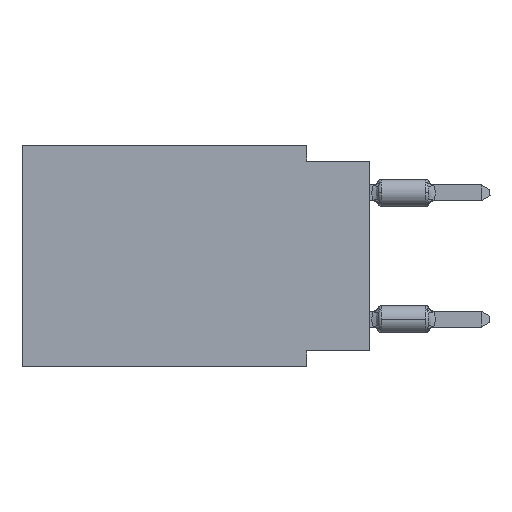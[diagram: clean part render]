
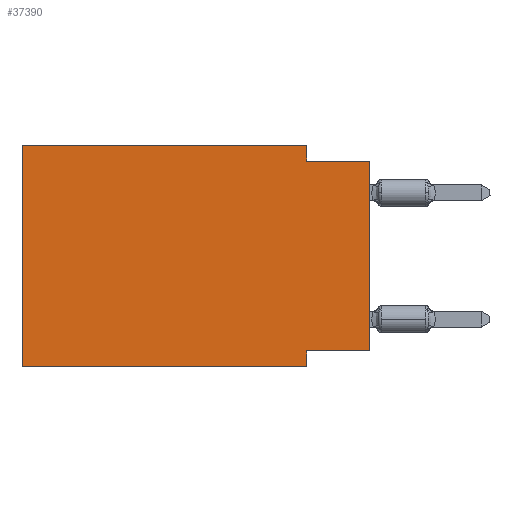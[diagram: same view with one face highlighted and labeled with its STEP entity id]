
A CAD part, left-side view. The second image highlights one B-rep face of the part: STEP entity #37390.
In plain terms, the highlighted planar face has unit normal (-1, 0, 0).
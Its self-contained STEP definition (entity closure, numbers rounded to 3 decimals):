
#150 = CARTESIAN_POINT ( 'NONE',  ( 0., 13.97, 0. ) ) ;
#561 = LINE ( 'NONE', #11217, #10341 ) ;
#792 = DIRECTION ( 'NONE',  ( 0., 0., -1. ) ) ;
#1008 = VERTEX_POINT ( 'NONE', #30699 ) ;
#1173 = DIRECTION ( 'NONE',  ( 0., 0., -1. ) ) ;
#2580 = LINE ( 'NONE', #2829, #40246 ) ;
#2829 = CARTESIAN_POINT ( 'NONE',  ( 0., 13.97, 0. ) ) ;
#3080 = ORIENTED_EDGE ( 'NONE', *, *, #45692, .F. ) ;
#5302 = CARTESIAN_POINT ( 'NONE',  ( 0., 0., 0. ) ) ;
#5452 = ORIENTED_EDGE ( 'NONE', *, *, #14774, .F. ) ;
#6140 = ORIENTED_EDGE ( 'NONE', *, *, #12411, .F. ) ;
#8449 = VECTOR ( 'NONE', #9900, 1000. ) ;
#8931 = AXIS2_PLACEMENT_3D ( 'NONE', #49040, #38356, #45553 ) ;
#9270 = LINE ( 'NONE', #20926, #18424 ) ;
#9900 = DIRECTION ( 'NONE',  ( 0., -1., 0. ) ) ;
#10341 = VECTOR ( 'NONE', #792, 1000. ) ;
#11217 = CARTESIAN_POINT ( 'NONE',  ( 0., 2.54, -8.89 ) ) ;
#12357 = LINE ( 'NONE', #23748, #25128 ) ;
#12411 = EDGE_CURVE ( 'NONE', #19675, #39759, #42293, .T. ) ;
#13213 = VERTEX_POINT ( 'NONE', #41444 ) ;
#13429 = VECTOR ( 'NONE', #1173, 1000. ) ;
#14661 = EDGE_CURVE ( 'NONE', #21927, #38828, #38777, .T. ) ;
#14774 = EDGE_CURVE ( 'NONE', #21927, #41085, #9270, .T. ) ;
#15375 = ORIENTED_EDGE ( 'NONE', *, *, #14661, .T. ) ;
#17890 = CARTESIAN_POINT ( 'NONE',  ( 0., 13.97, 0. ) ) ;
#18424 = VECTOR ( 'NONE', #43947, 1000. ) ;
#18802 = FACE_OUTER_BOUND ( 'NONE', #39040, .T. ) ;
#19052 = ORIENTED_EDGE ( 'NONE', *, *, #45977, .T. ) ;
#19507 = ORIENTED_EDGE ( 'NONE', *, *, #26186, .F. ) ;
#19675 = VERTEX_POINT ( 'NONE', #17890 ) ;
#20926 = CARTESIAN_POINT ( 'NONE',  ( 0., 0., -8.255 ) ) ;
#21653 = CARTESIAN_POINT ( 'NONE',  ( 0., 0., -0.635 ) ) ;
#21927 = VERTEX_POINT ( 'NONE', #41802 ) ;
#23737 = LINE ( 'NONE', #38854, #13429 ) ;
#23748 = CARTESIAN_POINT ( 'NONE',  ( 0., 13.97, -8.89 ) ) ;
#25128 = VECTOR ( 'NONE', #30941, 1000. ) ;
#26145 = VECTOR ( 'NONE', #26931, 1000. ) ;
#26186 = EDGE_CURVE ( 'NONE', #13213, #19675, #2580, .T. ) ;
#26931 = DIRECTION ( 'NONE',  ( 0., -1., 0. ) ) ;
#27170 = EDGE_CURVE ( 'NONE', #41085, #1008, #561, .T. ) ;
#27893 = ORIENTED_EDGE ( 'NONE', *, *, #28112, .F. ) ;
#28112 = EDGE_CURVE ( 'NONE', #39759, #28387, #23737, .T. ) ;
#28387 = VERTEX_POINT ( 'NONE', #45194 ) ;
#30433 = PLANE ( 'NONE',  #8931 ) ;
#30699 = CARTESIAN_POINT ( 'NONE',  ( 0., 2.54, -8.89 ) ) ;
#30941 = DIRECTION ( 'NONE',  ( 0., -1., 0. ) ) ;
#36132 = ORIENTED_EDGE ( 'NONE', *, *, #27170, .F. ) ;
#36183 = LINE ( 'NONE', #47100, #8449 ) ;
#37390 = ADVANCED_FACE ( 'NONE', ( #18802 ), #30433, .F. ) ;
#38356 = DIRECTION ( 'NONE',  ( 1., 0., 0. ) ) ;
#38777 = LINE ( 'NONE', #5302, #41313 ) ;
#38828 = VERTEX_POINT ( 'NONE', #21653 ) ;
#38854 = CARTESIAN_POINT ( 'NONE',  ( 0., 2.54, 0. ) ) ;
#39040 = EDGE_LOOP ( 'NONE', ( #15375, #3080, #27893, #6140, #19507, #19052, #36132, #5452 ) ) ;
#39759 = VERTEX_POINT ( 'NONE', #40124 ) ;
#40124 = CARTESIAN_POINT ( 'NONE',  ( 0., 2.54, 0. ) ) ;
#40246 = VECTOR ( 'NONE', #48214, 1000. ) ;
#41085 = VERTEX_POINT ( 'NONE', #45062 ) ;
#41313 = VECTOR ( 'NONE', #42004, 1000. ) ;
#41444 = CARTESIAN_POINT ( 'NONE',  ( 0., 13.97, -8.89 ) ) ;
#41802 = CARTESIAN_POINT ( 'NONE',  ( 0., 0., -8.255 ) ) ;
#42004 = DIRECTION ( 'NONE',  ( 0., 0., 1. ) ) ;
#42293 = LINE ( 'NONE', #150, #26145 ) ;
#43947 = DIRECTION ( 'NONE',  ( 0., 1., 0. ) ) ;
#45062 = CARTESIAN_POINT ( 'NONE',  ( 0., 2.54, -8.255 ) ) ;
#45194 = CARTESIAN_POINT ( 'NONE',  ( 0., 2.54, -0.635 ) ) ;
#45553 = DIRECTION ( 'NONE',  ( 0., 0., -1. ) ) ;
#45692 = EDGE_CURVE ( 'NONE', #28387, #38828, #36183, .T. ) ;
#45977 = EDGE_CURVE ( 'NONE', #13213, #1008, #12357, .T. ) ;
#47100 = CARTESIAN_POINT ( 'NONE',  ( 0., 0., -0.635 ) ) ;
#48214 = DIRECTION ( 'NONE',  ( 0., 0., 1. ) ) ;
#49040 = CARTESIAN_POINT ( 'NONE',  ( 0., 13.97, 0. ) ) ;
